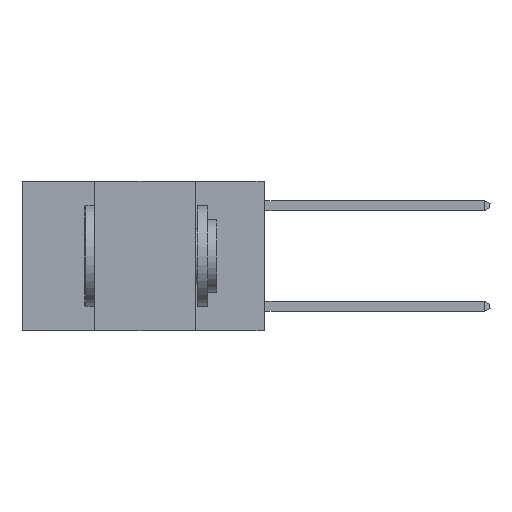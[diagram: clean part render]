
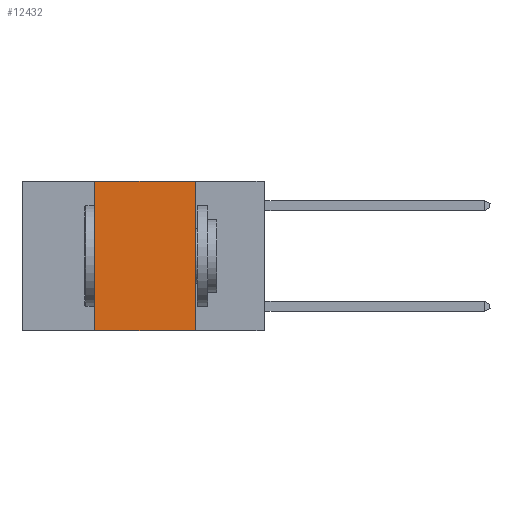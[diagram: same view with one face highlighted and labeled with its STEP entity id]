
A CAD part, left-side view. The second image highlights one B-rep face of the part: STEP entity #12432.
In plain terms, the highlighted planar face has unit normal (-1, 0, 0).
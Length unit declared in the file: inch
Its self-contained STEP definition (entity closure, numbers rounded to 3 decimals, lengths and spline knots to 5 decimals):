
#479 = VERTEX_POINT ( 'NONE', #19435 ) ;
#1567 = DIRECTION ( 'NONE',  ( 1., 0., 0. ) ) ;
#2168 = ORIENTED_EDGE ( 'NONE', *, *, #19536, .T. ) ;
#2270 = EDGE_CURVE ( 'NONE', #479, #6108, #14040, .T. ) ;
#2786 = ORIENTED_EDGE ( 'NONE', *, *, #2270, .F. ) ;
#3640 = CARTESIAN_POINT ( 'NONE',  ( 0., 0.6, 0. ) ) ;
#3849 = LINE ( 'NONE', #7126, #14035 ) ;
#4109 = CARTESIAN_POINT ( 'NONE',  ( 0., 0.42, 0. ) ) ;
#6108 = VERTEX_POINT ( 'NONE', #12548 ) ;
#7126 = CARTESIAN_POINT ( 'NONE',  ( 0., 0.42, 0. ) ) ;
#7150 = LINE ( 'NONE', #10682, #16842 ) ;
#7581 = LINE ( 'NONE', #22396, #9328 ) ;
#8361 = DIRECTION ( 'NONE',  ( 0., 0., -1. ) ) ;
#8415 = ORIENTED_EDGE ( 'NONE', *, *, #23871, .F. ) ;
#8885 = PLANE ( 'NONE',  #17639 ) ;
#8934 = VECTOR ( 'NONE', #8361, 39.37008 ) ;
#9328 = VECTOR ( 'NONE', #18514, 39.37008 ) ;
#10682 = CARTESIAN_POINT ( 'NONE',  ( 0., 0.6, 0. ) ) ;
#12133 = EDGE_LOOP ( 'NONE', ( #2786, #8415, #16601, #2168 ) ) ;
#12432 = ADVANCED_FACE ( 'NONE', ( #20280 ), #8885, .F. ) ;
#12548 = CARTESIAN_POINT ( 'NONE',  ( 0., 0.17, -0.37 ) ) ;
#14035 = VECTOR ( 'NONE', #21828, 39.37008 ) ;
#14040 = LINE ( 'NONE', #21600, #8934 ) ;
#15081 = VERTEX_POINT ( 'NONE', #4109 ) ;
#16601 = ORIENTED_EDGE ( 'NONE', *, *, #22307, .F. ) ;
#16842 = VECTOR ( 'NONE', #19774, 39.37008 ) ;
#17639 = AXIS2_PLACEMENT_3D ( 'NONE', #3640, #1567, #20157 ) ;
#18514 = DIRECTION ( 'NONE',  ( 0., -1., 0. ) ) ;
#19435 = CARTESIAN_POINT ( 'NONE',  ( 0., 0.17, 0. ) ) ;
#19465 = CARTESIAN_POINT ( 'NONE',  ( 0., 0.42, -0.37 ) ) ;
#19536 = EDGE_CURVE ( 'NONE', #23015, #6108, #7581, .T. ) ;
#19774 = DIRECTION ( 'NONE',  ( 0., -1., 0. ) ) ;
#20157 = DIRECTION ( 'NONE',  ( 0., 0., -1. ) ) ;
#20280 = FACE_OUTER_BOUND ( 'NONE', #12133, .T. ) ;
#21600 = CARTESIAN_POINT ( 'NONE',  ( 0., 0.17, 0. ) ) ;
#21828 = DIRECTION ( 'NONE',  ( 0., 0., 1. ) ) ;
#22307 = EDGE_CURVE ( 'NONE', #23015, #15081, #3849, .T. ) ;
#22396 = CARTESIAN_POINT ( 'NONE',  ( 0., 0.6, -0.37 ) ) ;
#23015 = VERTEX_POINT ( 'NONE', #19465 ) ;
#23871 = EDGE_CURVE ( 'NONE', #15081, #479, #7150, .T. ) ;
